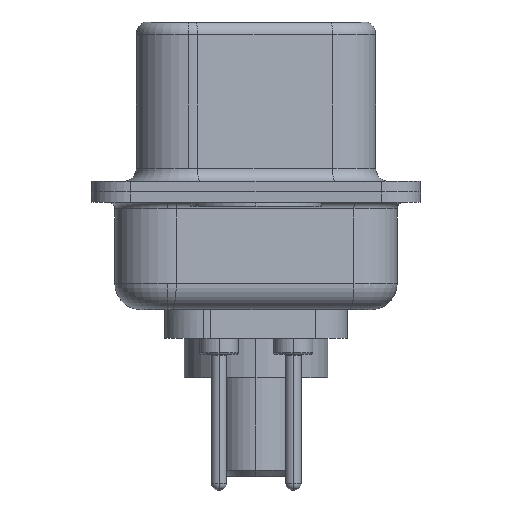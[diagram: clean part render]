
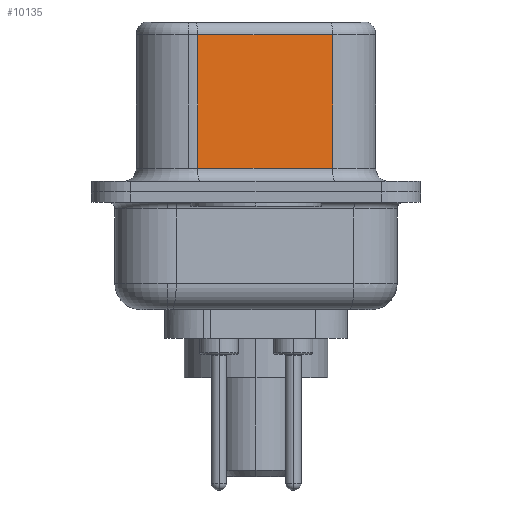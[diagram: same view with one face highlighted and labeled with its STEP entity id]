
A CAD part, left-side view. The second image highlights one B-rep face of the part: STEP entity #10135.
In plain terms, the highlighted planar face has unit normal (-0.985, -0.174, 0).
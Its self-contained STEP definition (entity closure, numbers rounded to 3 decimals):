
#178 = VERTEX_POINT ( 'NONE', #2544 ) ;
#181 = DIRECTION ( 'NONE',  ( -0.174, 0.985, 0. ) ) ;
#359 = DIRECTION ( 'NONE',  ( 0.985, 0.174, 0. ) ) ;
#610 = ORIENTED_EDGE ( 'NONE', *, *, #6376, .F. ) ;
#651 = EDGE_LOOP ( 'NONE', ( #610, #6108, #11764, #4220 ) ) ;
#652 = LINE ( 'NONE', #5356, #2991 ) ;
#950 = VERTEX_POINT ( 'NONE', #4990 ) ;
#1270 = CARTESIAN_POINT ( 'NONE',  ( 4.58, -2.927, 6.52 ) ) ;
#1684 = DIRECTION ( 'NONE',  ( 0., 0., -1. ) ) ;
#2280 = CARTESIAN_POINT ( 'NONE',  ( 4.58, -2.927, 0.9 ) ) ;
#2422 = DIRECTION ( 'NONE',  ( 0.174, -0.985, 0. ) ) ;
#2466 = PLANE ( 'NONE',  #8763 ) ;
#2544 = CARTESIAN_POINT ( 'NONE',  ( 3.67, 2.233, 6.02 ) ) ;
#2835 = VECTOR ( 'NONE', #11795, 1000. ) ;
#2991 = VECTOR ( 'NONE', #7410, 1000. ) ;
#3932 = CARTESIAN_POINT ( 'NONE',  ( 3.67, 2.233, 0.9 ) ) ;
#4075 = VECTOR ( 'NONE', #1684, 1000. ) ;
#4220 = ORIENTED_EDGE ( 'NONE', *, *, #7808, .T. ) ;
#4990 = CARTESIAN_POINT ( 'NONE',  ( 4.58, -2.927, 6.02 ) ) ;
#5158 = FACE_OUTER_BOUND ( 'NONE', #651, .T. ) ;
#5338 = VERTEX_POINT ( 'NONE', #3932 ) ;
#5350 = EDGE_CURVE ( 'NONE', #950, #178, #652, .T. ) ;
#5356 = CARTESIAN_POINT ( 'NONE',  ( 4.58, -2.927, 6.02 ) ) ;
#5575 = VECTOR ( 'NONE', #2422, 1000. ) ;
#6108 = ORIENTED_EDGE ( 'NONE', *, *, #5350, .T. ) ;
#6376 = EDGE_CURVE ( 'NONE', #950, #11612, #12097, .T. ) ;
#7410 = DIRECTION ( 'NONE',  ( -0.174, 0.985, 0. ) ) ;
#7660 = CARTESIAN_POINT ( 'NONE',  ( 4.58, -2.927, 6.52 ) ) ;
#7808 = EDGE_CURVE ( 'NONE', #5338, #11612, #8271, .T. ) ;
#8049 = EDGE_CURVE ( 'NONE', #178, #5338, #9563, .T. ) ;
#8199 = CARTESIAN_POINT ( 'NONE',  ( 3.67, 2.233, 6.52 ) ) ;
#8271 = LINE ( 'NONE', #2280, #5575 ) ;
#8763 = AXIS2_PLACEMENT_3D ( 'NONE', #1270, #359, #181 ) ;
#9563 = LINE ( 'NONE', #8199, #4075 ) ;
#10135 = ADVANCED_FACE ( 'NONE', ( #5158 ), #2466, .F. ) ;
#10561 = CARTESIAN_POINT ( 'NONE',  ( 4.58, -2.927, 0.9 ) ) ;
#11612 = VERTEX_POINT ( 'NONE', #10561 ) ;
#11764 = ORIENTED_EDGE ( 'NONE', *, *, #8049, .T. ) ;
#11795 = DIRECTION ( 'NONE',  ( 0., 0., -1. ) ) ;
#12097 = LINE ( 'NONE', #7660, #2835 ) ;
